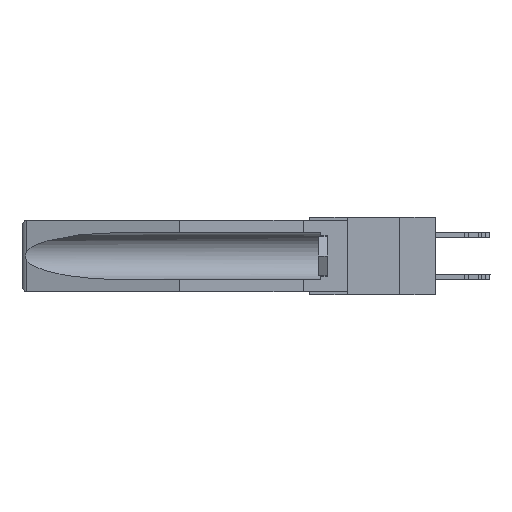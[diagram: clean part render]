
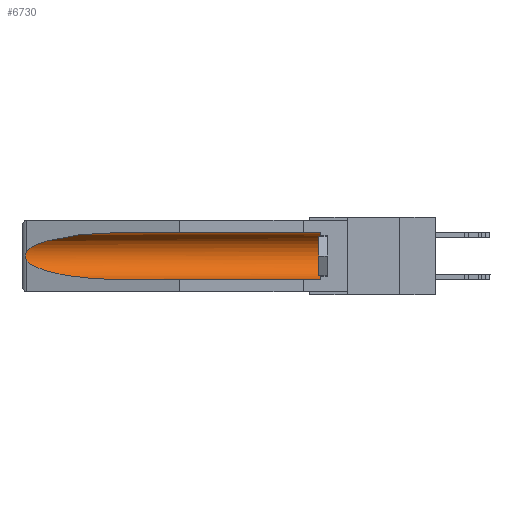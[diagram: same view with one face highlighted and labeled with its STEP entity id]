
A CAD part, left-side view. The second image highlights one B-rep face of the part: STEP entity #6730.
In plain terms, the highlighted cylindrical face has radius 2.857 mm (diameter 5.715 mm), a partial arc.
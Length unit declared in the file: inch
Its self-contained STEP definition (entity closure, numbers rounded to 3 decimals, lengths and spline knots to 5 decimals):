
#253 =( BOUNDED_CURVE ( )  B_SPLINE_CURVE ( 3, ( #33804, #15342, #9863, #7773 ),
 .UNSPECIFIED., .F., .T. ) 
 B_SPLINE_CURVE_WITH_KNOTS ( ( 4, 4 ),
 ( 4.71239, 6.08839 ),
 .UNSPECIFIED. ) 
 CURVE ( )  GEOMETRIC_REPRESENTATION_ITEM ( )  RATIONAL_B_SPLINE_CURVE ( ( 1., 0.848, 0.848, 1. ) ) 
 REPRESENTATION_ITEM ( '' )  );
#1179 = EDGE_CURVE ( 'NONE', #28681, #25641, #6279, .T. ) ;
#1766 = VERTEX_POINT ( 'NONE', #5460 ) ;
#1819 = ORIENTED_EDGE ( 'NONE', *, *, #30117, .T. ) ;
#3980 = EDGE_CURVE ( 'NONE', #5623, #13672, #11346, .T. ) ;
#4219 = CARTESIAN_POINT ( 'NONE',  ( 0.2675, 1.53308, -0.16763 ) ) ;
#4650 = CARTESIAN_POINT ( 'NONE',  ( 0.155, -0.30754, -0.1715 ) ) ;
#5460 = CARTESIAN_POINT ( 'NONE',  ( 0.155, 1.07973, -0.059 ) ) ;
#5623 = VERTEX_POINT ( 'NONE', #5844 ) ;
#5844 = CARTESIAN_POINT ( 'NONE',  ( 0.26537, 1.52718, -0.19328 ) ) ;
#5975 = VECTOR ( 'NONE', #7578, 39.37008 ) ;
#6279 = CIRCLE ( 'NONE', #26671, 0.1125 ) ;
#6730 = ADVANCED_FACE ( 'NONE', ( #15884 ), #24063, .F. ) ;
#6752 = CARTESIAN_POINT ( 'NONE',  ( 0.25451, 1.48313, -0.24835 ) ) ;
#6859 = CARTESIAN_POINT ( 'NONE',  ( 0.155, 1.07973, -0.284 ) ) ;
#7578 = DIRECTION ( 'NONE',  ( 0., 1., 0. ) ) ;
#7688 = DIRECTION ( 'NONE',  ( 0., 0., 1. ) ) ;
#7773 = CARTESIAN_POINT ( 'NONE',  ( 0.26537, 1.52718, -0.14972 ) ) ;
#8201 = EDGE_CURVE ( 'NONE', #25641, #1766, #31661, .T. ) ;
#9151 = CARTESIAN_POINT ( 'NONE',  ( 0.26597, 1.52961, -0.15275 ) ) ;
#9161 = CARTESIAN_POINT ( 'NONE',  ( 0.21114, 1.30732, -0.284 ) ) ;
#9224 = ORIENTED_EDGE ( 'NONE', *, *, #9990, .F. ) ;
#9582 = CARTESIAN_POINT ( 'NONE',  ( 0.155, 0.126, -0.284 ) ) ;
#9863 = CARTESIAN_POINT ( 'NONE',  ( 0.25451, 1.48313, -0.09465 ) ) ;
#9990 = EDGE_CURVE ( 'NONE', #28681, #13672, #30486, .T. ) ;
#11346 =( BOUNDED_CURVE ( )  B_SPLINE_CURVE ( 3, ( #22504, #6752, #9161, #6859 ),
 .UNSPECIFIED., .F., .F. ) 
 B_SPLINE_CURVE_WITH_KNOTS ( ( 4, 4 ),
 ( 0.1948, 1.5708 ),
 .UNSPECIFIED. ) 
 CURVE ( )  GEOMETRIC_REPRESENTATION_ITEM ( )  RATIONAL_B_SPLINE_CURVE ( ( 1., 0.848, 0.848, 1. ) ) 
 REPRESENTATION_ITEM ( '' )  );
#13398 = CARTESIAN_POINT ( 'NONE',  ( 0.155, 1.07973, -0.284 ) ) ;
#13672 = VERTEX_POINT ( 'NONE', #13398 ) ;
#14406 = CARTESIAN_POINT ( 'NONE',  ( 0.2675, 1.53308, -0.17534 ) ) ;
#15342 = CARTESIAN_POINT ( 'NONE',  ( 0.21114, 1.30732, -0.059 ) ) ;
#15861 = ORIENTED_EDGE ( 'NONE', *, *, #21611, .T. ) ;
#15884 = FACE_OUTER_BOUND ( 'NONE', #19744, .T. ) ;
#16783 = CARTESIAN_POINT ( 'NONE',  ( 0.2673, 1.5327, -0.16383 ) ) ;
#17121 = CARTESIAN_POINT ( 'NONE',  ( 0.26537, 1.52718, -0.19328 ) ) ;
#17513 = ORIENTED_EDGE ( 'NONE', *, *, #1179, .T. ) ;
#17726 = DIRECTION ( 'NONE',  ( 0., -1., 0. ) ) ;
#17808 = CARTESIAN_POINT ( 'NONE',  ( 0.26537, 1.52718, -0.14972 ) ) ;
#19040 = CARTESIAN_POINT ( 'NONE',  ( 0.155, 0.126, -0.059 ) ) ;
#19434 = VECTOR ( 'NONE', #19758, 39.37008 ) ;
#19744 = EDGE_LOOP ( 'NONE', ( #1819, #15861, #21002, #9224, #17513, #26084 ) ) ;
#19758 = DIRECTION ( 'NONE',  ( 0., 1., 0. ) ) ;
#20484 = CARTESIAN_POINT ( 'NONE',  ( 0.155, 0.126, -0.1715 ) ) ;
#21002 = ORIENTED_EDGE ( 'NONE', *, *, #3980, .T. ) ;
#21611 = EDGE_CURVE ( 'NONE', #30143, #5623, #24972, .T. ) ;
#22029 = CARTESIAN_POINT ( 'NONE',  ( 0.26655, 1.53094, -0.18657 ) ) ;
#22504 = CARTESIAN_POINT ( 'NONE',  ( 0.26537, 1.52718, -0.19328 ) ) ;
#24063 = CYLINDRICAL_SURFACE ( 'NONE', #26327, 0.1125 ) ;
#24747 = DIRECTION ( 'NONE',  ( 0., 0., 1. ) ) ;
#24972 = B_SPLINE_CURVE_WITH_KNOTS ( 'NONE', 3,
 ( #27387, #9151, #32519, #16783, #4219, #14406, #30124, #22029, #32748, #17121 ),
 .UNSPECIFIED., .F., .F.,
 ( 4, 2, 2, 2, 4 ),
 ( 0., 0.00029, 0.00058, 0.00087, 0.00117 ),
 .UNSPECIFIED. ) ;
#25641 = VERTEX_POINT ( 'NONE', #19040 ) ;
#26084 = ORIENTED_EDGE ( 'NONE', *, *, #8201, .T. ) ;
#26327 = AXIS2_PLACEMENT_3D ( 'NONE', #4650, #30426, #24747 ) ;
#26671 = AXIS2_PLACEMENT_3D ( 'NONE', #20484, #17726, #7688 ) ;
#27387 = CARTESIAN_POINT ( 'NONE',  ( 0.26537, 1.52718, -0.14972 ) ) ;
#28681 = VERTEX_POINT ( 'NONE', #9582 ) ;
#30117 = EDGE_CURVE ( 'NONE', #1766, #30143, #253, .T. ) ;
#30124 = CARTESIAN_POINT ( 'NONE',  ( 0.2673, 1.53269, -0.17917 ) ) ;
#30143 = VERTEX_POINT ( 'NONE', #17808 ) ;
#30426 = DIRECTION ( 'NONE',  ( 0., 1., 0. ) ) ;
#30486 = LINE ( 'NONE', #31068, #5975 ) ;
#31068 = CARTESIAN_POINT ( 'NONE',  ( 0.155, -0.30754, -0.284 ) ) ;
#31661 = LINE ( 'NONE', #32537, #19434 ) ;
#32519 = CARTESIAN_POINT ( 'NONE',  ( 0.26654, 1.53092, -0.15636 ) ) ;
#32537 = CARTESIAN_POINT ( 'NONE',  ( 0.155, -0.30754, -0.059 ) ) ;
#32748 = CARTESIAN_POINT ( 'NONE',  ( 0.26597, 1.5296, -0.19026 ) ) ;
#33804 = CARTESIAN_POINT ( 'NONE',  ( 0.155, 1.07973, -0.059 ) ) ;
